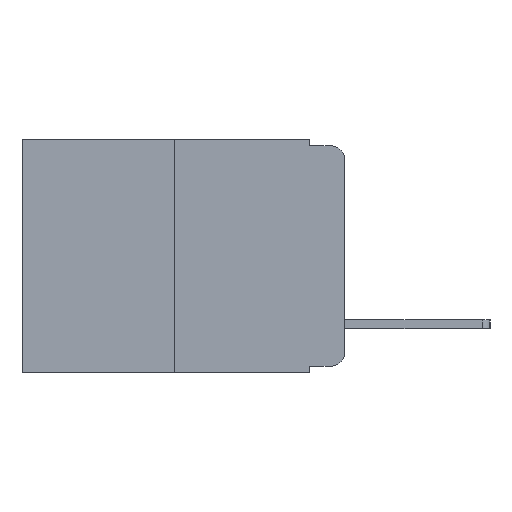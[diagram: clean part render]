
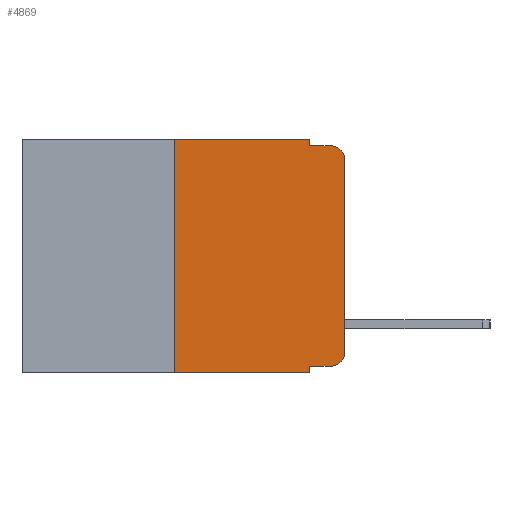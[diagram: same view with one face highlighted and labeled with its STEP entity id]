
A CAD part, left-side view. The second image highlights one B-rep face of the part: STEP entity #4869.
In plain terms, the highlighted planar face has unit normal (-1, 0, 0).
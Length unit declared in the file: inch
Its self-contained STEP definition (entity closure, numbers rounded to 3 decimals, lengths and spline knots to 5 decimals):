
#169 = LINE ( 'NONE', #2103, #9863 ) ;
#229 = EDGE_CURVE ( 'NONE', #8168, #2301, #10363, .T. ) ;
#412 = CARTESIAN_POINT ( 'NONE',  ( 0., 0.25, 0. ) ) ;
#521 = CARTESIAN_POINT ( 'NONE',  ( 0., 0., -0.03 ) ) ;
#571 = CARTESIAN_POINT ( 'NONE',  ( 0., 0.051, -0.333 ) ) ;
#955 = VERTEX_POINT ( 'NONE', #9217 ) ;
#1116 = CARTESIAN_POINT ( 'NONE',  ( 0., 0.473, 0. ) ) ;
#1138 = DIRECTION ( 'NONE',  ( 0., 0., -1. ) ) ;
#1159 = CIRCLE ( 'NONE', #6864, 0.02 ) ;
#1284 = CARTESIAN_POINT ( 'NONE',  ( 0., 0.051, -0.343 ) ) ;
#1591 = DIRECTION ( 'NONE',  ( -1., 0., 0. ) ) ;
#1825 = VECTOR ( 'NONE', #1896, 39.37008 ) ;
#1896 = DIRECTION ( 'NONE',  ( 0., -1., 0. ) ) ;
#1946 = CARTESIAN_POINT ( 'NONE',  ( 0., 0.02, -0.03 ) ) ;
#2103 = CARTESIAN_POINT ( 'NONE',  ( 0., 0.473, -0.343 ) ) ;
#2301 = VERTEX_POINT ( 'NONE', #412 ) ;
#2362 = CARTESIAN_POINT ( 'NONE',  ( 0., 0.051, 0. ) ) ;
#2377 = CARTESIAN_POINT ( 'NONE',  ( 0., 0.051, -0.01 ) ) ;
#2590 = CARTESIAN_POINT ( 'NONE',  ( 0., 0.051, -0.333 ) ) ;
#2653 = LINE ( 'NONE', #2362, #6047 ) ;
#2909 = EDGE_CURVE ( 'NONE', #955, #4543, #9325, .T. ) ;
#3286 = DIRECTION ( 'NONE',  ( 0., 0., -1. ) ) ;
#3618 = PLANE ( 'NONE',  #6737 ) ;
#3856 = VECTOR ( 'NONE', #13501, 39.37008 ) ;
#3929 = CIRCLE ( 'NONE', #14464, 0.02 ) ;
#4543 = VERTEX_POINT ( 'NONE', #8847 ) ;
#4575 = DIRECTION ( 'NONE',  ( 0., -1., 0. ) ) ;
#4869 = ADVANCED_FACE ( 'NONE', ( #14563 ), #3618, .F. ) ;
#5078 = VERTEX_POINT ( 'NONE', #10052 ) ;
#5732 = ORIENTED_EDGE ( 'NONE', *, *, #9553, .T. ) ;
#5758 = ORIENTED_EDGE ( 'NONE', *, *, #6339, .F. ) ;
#5876 = ORIENTED_EDGE ( 'NONE', *, *, #229, .F. ) ;
#5901 = ORIENTED_EDGE ( 'NONE', *, *, #13453, .F. ) ;
#5919 = ORIENTED_EDGE ( 'NONE', *, *, #7354, .T. ) ;
#5979 = ORIENTED_EDGE ( 'NONE', *, *, #8748, .T. ) ;
#6047 = VECTOR ( 'NONE', #8594, 39.37008 ) ;
#6106 = ORIENTED_EDGE ( 'NONE', *, *, #14697, .F. ) ;
#6119 = VERTEX_POINT ( 'NONE', #13900 ) ;
#6136 = ORIENTED_EDGE ( 'NONE', *, *, #13124, .T. ) ;
#6145 = ORIENTED_EDGE ( 'NONE', *, *, #13935, .T. ) ;
#6339 = EDGE_CURVE ( 'NONE', #4543, #6119, #15038, .T. ) ;
#6381 = CARTESIAN_POINT ( 'NONE',  ( 0., 0., 0. ) ) ;
#6737 = AXIS2_PLACEMENT_3D ( 'NONE', #1116, #7095, #1138 ) ;
#6864 = AXIS2_PLACEMENT_3D ( 'NONE', #1946, #10650, #3286 ) ;
#7095 = DIRECTION ( 'NONE',  ( 1., 0., 0. ) ) ;
#7354 = EDGE_CURVE ( 'NONE', #8168, #7837, #169, .T. ) ;
#7546 = DIRECTION ( 'NONE',  ( 0., 0., 1. ) ) ;
#7837 = VERTEX_POINT ( 'NONE', #1284 ) ;
#8133 = VERTEX_POINT ( 'NONE', #521 ) ;
#8168 = VERTEX_POINT ( 'NONE', #14220 ) ;
#8177 = VERTEX_POINT ( 'NONE', #15449 ) ;
#8594 = DIRECTION ( 'NONE',  ( 0., 0., -1. ) ) ;
#8748 = EDGE_CURVE ( 'NONE', #8133, #6119, #1159, .T. ) ;
#8847 = CARTESIAN_POINT ( 'NONE',  ( 0., 0.051, -0.01 ) ) ;
#8904 = LINE ( 'NONE', #571, #1825 ) ;
#9032 = VECTOR ( 'NONE', #7546, 39.37008 ) ;
#9119 = CARTESIAN_POINT ( 'NONE',  ( 0., 0.02, -0.313 ) ) ;
#9217 = CARTESIAN_POINT ( 'NONE',  ( 0., 0.051, 0. ) ) ;
#9325 = LINE ( 'NONE', #13882, #12574 ) ;
#9553 = EDGE_CURVE ( 'NONE', #5078, #8133, #11886, .T. ) ;
#9580 = VERTEX_POINT ( 'NONE', #2590 ) ;
#9802 = DIRECTION ( 'NONE',  ( 0., 0., -1. ) ) ;
#9863 = VECTOR ( 'NONE', #13628, 39.37008 ) ;
#10052 = CARTESIAN_POINT ( 'NONE',  ( 0., 0., -0.313 ) ) ;
#10322 = DIRECTION ( 'NONE',  ( 0., 0., -1. ) ) ;
#10363 = LINE ( 'NONE', #13384, #3856 ) ;
#10650 = DIRECTION ( 'NONE',  ( -1., 0., 0. ) ) ;
#11275 = ORIENTED_EDGE ( 'NONE', *, *, #2909, .F. ) ;
#11886 = LINE ( 'NONE', #6381, #9032 ) ;
#12547 = VECTOR ( 'NONE', #15706, 39.37008 ) ;
#12574 = VECTOR ( 'NONE', #9802, 39.37008 ) ;
#13124 = EDGE_CURVE ( 'NONE', #8177, #5078, #3929, .T. ) ;
#13384 = CARTESIAN_POINT ( 'NONE',  ( 0., 0.25, 0. ) ) ;
#13453 = EDGE_CURVE ( 'NONE', #2301, #955, #15629, .T. ) ;
#13501 = DIRECTION ( 'NONE',  ( 0., 0., 1. ) ) ;
#13628 = DIRECTION ( 'NONE',  ( 0., -1., 0. ) ) ;
#13882 = CARTESIAN_POINT ( 'NONE',  ( 0., 0.051, 0. ) ) ;
#13883 = EDGE_LOOP ( 'NONE', ( #5732, #5979, #5758, #11275, #5901, #5876, #5919, #6106, #6145, #6136 ) ) ;
#13900 = CARTESIAN_POINT ( 'NONE',  ( 0., 0.02, -0.01 ) ) ;
#13935 = EDGE_CURVE ( 'NONE', #9580, #8177, #8904, .T. ) ;
#14220 = CARTESIAN_POINT ( 'NONE',  ( 0., 0.25, -0.343 ) ) ;
#14464 = AXIS2_PLACEMENT_3D ( 'NONE', #9119, #1591, #10322 ) ;
#14563 = FACE_OUTER_BOUND ( 'NONE', #13883, .T. ) ;
#14583 = CARTESIAN_POINT ( 'NONE',  ( 0., 0.473, 0. ) ) ;
#14693 = VECTOR ( 'NONE', #4575, 39.37008 ) ;
#14697 = EDGE_CURVE ( 'NONE', #9580, #7837, #2653, .T. ) ;
#15038 = LINE ( 'NONE', #2377, #14693 ) ;
#15449 = CARTESIAN_POINT ( 'NONE',  ( 0., 0.02, -0.333 ) ) ;
#15629 = LINE ( 'NONE', #14583, #12547 ) ;
#15706 = DIRECTION ( 'NONE',  ( 0., -1., 0. ) ) ;
